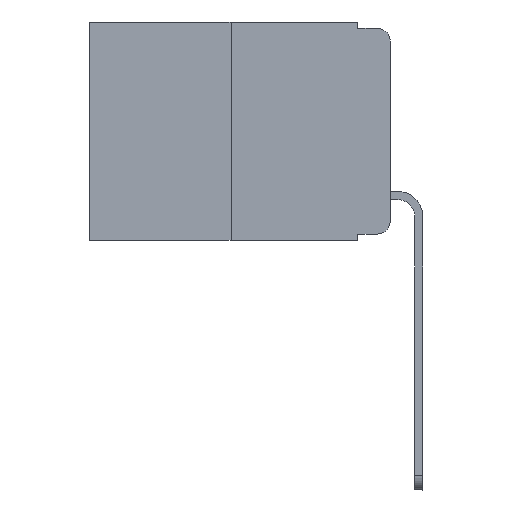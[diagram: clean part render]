
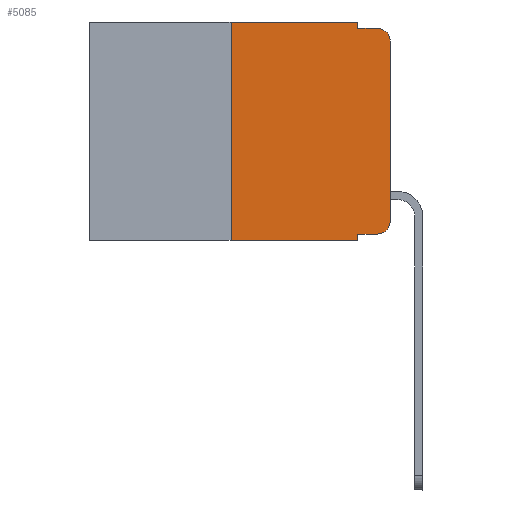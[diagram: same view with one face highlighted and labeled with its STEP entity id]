
A CAD part, left-side view. The second image highlights one B-rep face of the part: STEP entity #5085.
In plain terms, the highlighted planar face has unit normal (-1, 0, 0).
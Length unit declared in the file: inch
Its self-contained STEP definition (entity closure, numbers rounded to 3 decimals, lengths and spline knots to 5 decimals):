
#389 = CARTESIAN_POINT ( 'NONE',  ( 0., 0.051, 0. ) ) ;
#700 = LINE ( 'NONE', #18300, #17857 ) ;
#851 = EDGE_CURVE ( 'NONE', #16783, #2543, #10805, .T. ) ;
#1384 = CARTESIAN_POINT ( 'NONE',  ( 0., 0.25, 0. ) ) ;
#1413 = CIRCLE ( 'NONE', #5543, 0.02 ) ;
#1693 = VERTEX_POINT ( 'NONE', #14502 ) ;
#1701 = CARTESIAN_POINT ( 'NONE',  ( 0., 0.051, -0.01 ) ) ;
#1744 = CARTESIAN_POINT ( 'NONE',  ( 0., 0.051, -0.333 ) ) ;
#1804 = ORIENTED_EDGE ( 'NONE', *, *, #3738, .T. ) ;
#1873 = VERTEX_POINT ( 'NONE', #15319 ) ;
#2159 = DIRECTION ( 'NONE',  ( 0., 0., -1. ) ) ;
#2528 = DIRECTION ( 'NONE',  ( 1., 0., 0. ) ) ;
#2543 = VERTEX_POINT ( 'NONE', #22045 ) ;
#3181 = VERTEX_POINT ( 'NONE', #1744 ) ;
#3312 = ORIENTED_EDGE ( 'NONE', *, *, #7959, .T. ) ;
#3339 = VECTOR ( 'NONE', #2159, 39.37008 ) ;
#3738 = EDGE_CURVE ( 'NONE', #1693, #1873, #17899, .T. ) ;
#4029 = DIRECTION ( 'NONE',  ( -1., 0., 0. ) ) ;
#4048 = EDGE_CURVE ( 'NONE', #19154, #18996, #10962, .T. ) ;
#4309 = ORIENTED_EDGE ( 'NONE', *, *, #4048, .T. ) ;
#4413 = FACE_OUTER_BOUND ( 'NONE', #14501, .T. ) ;
#4692 = LINE ( 'NONE', #11640, #7896 ) ;
#5085 = ADVANCED_FACE ( 'NONE', ( #4413 ), #6068, .F. ) ;
#5519 = ORIENTED_EDGE ( 'NONE', *, *, #9241, .F. ) ;
#5543 = AXIS2_PLACEMENT_3D ( 'NONE', #20252, #4029, #18588 ) ;
#5679 = VERTEX_POINT ( 'NONE', #22838 ) ;
#6068 = PLANE ( 'NONE',  #7625 ) ;
#6938 = ORIENTED_EDGE ( 'NONE', *, *, #15785, .F. ) ;
#7316 = CARTESIAN_POINT ( 'NONE',  ( 0., 0.473, -0.343 ) ) ;
#7625 = AXIS2_PLACEMENT_3D ( 'NONE', #20512, #2528, #9725 ) ;
#7677 = DIRECTION ( 'NONE',  ( -1., 0., 0. ) ) ;
#7896 = VECTOR ( 'NONE', #18760, 39.37008 ) ;
#7959 = EDGE_CURVE ( 'NONE', #1873, #2543, #1413, .T. ) ;
#7971 = VERTEX_POINT ( 'NONE', #9593 ) ;
#9241 = EDGE_CURVE ( 'NONE', #3181, #18996, #9595, .T. ) ;
#9444 = EDGE_CURVE ( 'NONE', #19154, #15145, #14063, .T. ) ;
#9593 = CARTESIAN_POINT ( 'NONE',  ( 0., 0.051, 0. ) ) ;
#9595 = LINE ( 'NONE', #389, #3339 ) ;
#9695 = EDGE_CURVE ( 'NONE', #5679, #1693, #18447, .T. ) ;
#9725 = DIRECTION ( 'NONE',  ( 0., 0., -1. ) ) ;
#9877 = VECTOR ( 'NONE', #17681, 39.37008 ) ;
#10016 = ORIENTED_EDGE ( 'NONE', *, *, #10269, .F. ) ;
#10269 = EDGE_CURVE ( 'NONE', #7971, #16783, #4692, .T. ) ;
#10442 = DIRECTION ( 'NONE',  ( 0., 0., 1. ) ) ;
#10543 = ORIENTED_EDGE ( 'NONE', *, *, #9695, .T. ) ;
#10631 = EDGE_CURVE ( 'NONE', #3181, #5679, #12581, .T. ) ;
#10737 = CARTESIAN_POINT ( 'NONE',  ( 0., 0.25, 0. ) ) ;
#10805 = LINE ( 'NONE', #21361, #9877 ) ;
#10962 = LINE ( 'NONE', #7316, #13030 ) ;
#11203 = DIRECTION ( 'NONE',  ( 0., -1., 0. ) ) ;
#11640 = CARTESIAN_POINT ( 'NONE',  ( 0., 0.051, 0. ) ) ;
#12581 = LINE ( 'NONE', #12810, #18482 ) ;
#12810 = CARTESIAN_POINT ( 'NONE',  ( 0., 0.051, -0.333 ) ) ;
#13030 = VECTOR ( 'NONE', #23295, 39.37008 ) ;
#13522 = AXIS2_PLACEMENT_3D ( 'NONE', #16538, #7677, #14988 ) ;
#13858 = CARTESIAN_POINT ( 'NONE',  ( 0., 0.25, -0.343 ) ) ;
#14063 = LINE ( 'NONE', #10737, #20341 ) ;
#14175 = DIRECTION ( 'NONE',  ( 0., 0., 1. ) ) ;
#14501 = EDGE_LOOP ( 'NONE', ( #1804, #3312, #14870, #10016, #6938, #15050, #4309, #5519, #23160, #10543 ) ) ;
#14502 = CARTESIAN_POINT ( 'NONE',  ( 0., 0., -0.313 ) ) ;
#14870 = ORIENTED_EDGE ( 'NONE', *, *, #851, .F. ) ;
#14988 = DIRECTION ( 'NONE',  ( 0., 0., -1. ) ) ;
#15050 = ORIENTED_EDGE ( 'NONE', *, *, #9444, .F. ) ;
#15145 = VERTEX_POINT ( 'NONE', #1384 ) ;
#15319 = CARTESIAN_POINT ( 'NONE',  ( 0., 0., -0.03 ) ) ;
#15785 = EDGE_CURVE ( 'NONE', #15145, #7971, #700, .T. ) ;
#16283 = CARTESIAN_POINT ( 'NONE',  ( 0., 0.051, -0.343 ) ) ;
#16538 = CARTESIAN_POINT ( 'NONE',  ( 0., 0.02, -0.313 ) ) ;
#16783 = VERTEX_POINT ( 'NONE', #1701 ) ;
#17681 = DIRECTION ( 'NONE',  ( 0., -1., 0. ) ) ;
#17857 = VECTOR ( 'NONE', #11203, 39.37008 ) ;
#17899 = LINE ( 'NONE', #21692, #22440 ) ;
#18300 = CARTESIAN_POINT ( 'NONE',  ( 0., 0.473, 0. ) ) ;
#18447 = CIRCLE ( 'NONE', #13522, 0.02 ) ;
#18482 = VECTOR ( 'NONE', #20056, 39.37008 ) ;
#18588 = DIRECTION ( 'NONE',  ( 0., 0., -1. ) ) ;
#18760 = DIRECTION ( 'NONE',  ( 0., 0., -1. ) ) ;
#18996 = VERTEX_POINT ( 'NONE', #16283 ) ;
#19154 = VERTEX_POINT ( 'NONE', #13858 ) ;
#20056 = DIRECTION ( 'NONE',  ( 0., -1., 0. ) ) ;
#20252 = CARTESIAN_POINT ( 'NONE',  ( 0., 0.02, -0.03 ) ) ;
#20341 = VECTOR ( 'NONE', #14175, 39.37008 ) ;
#20512 = CARTESIAN_POINT ( 'NONE',  ( 0., 0.473, 0. ) ) ;
#21361 = CARTESIAN_POINT ( 'NONE',  ( 0., 0.051, -0.01 ) ) ;
#21692 = CARTESIAN_POINT ( 'NONE',  ( 0., 0., 0. ) ) ;
#22045 = CARTESIAN_POINT ( 'NONE',  ( 0., 0.02, -0.01 ) ) ;
#22440 = VECTOR ( 'NONE', #10442, 39.37008 ) ;
#22838 = CARTESIAN_POINT ( 'NONE',  ( 0., 0.02, -0.333 ) ) ;
#23160 = ORIENTED_EDGE ( 'NONE', *, *, #10631, .T. ) ;
#23295 = DIRECTION ( 'NONE',  ( 0., -1., 0. ) ) ;
